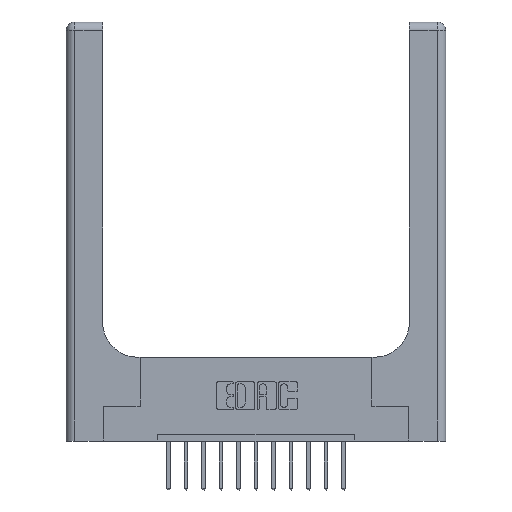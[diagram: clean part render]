
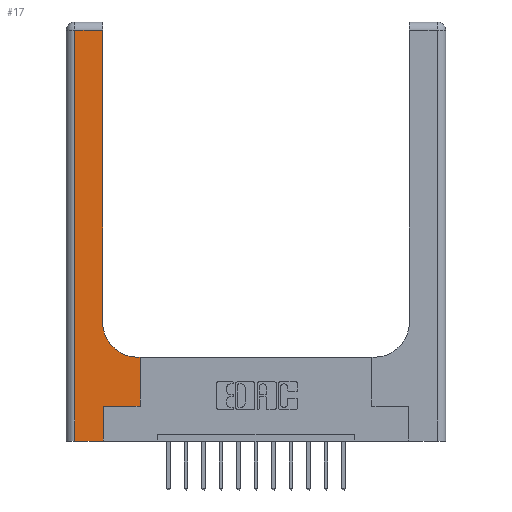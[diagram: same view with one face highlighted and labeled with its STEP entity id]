
A CAD part, top view. The second image highlights one B-rep face of the part: STEP entity #17.
In plain terms, the highlighted planar face has unit normal (0, 0, 1).
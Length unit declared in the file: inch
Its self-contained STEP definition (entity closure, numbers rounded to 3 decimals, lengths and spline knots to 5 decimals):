
#17 = ADVANCED_FACE ( 'NONE', ( #8297 ), #3548, .F. ) ;
#276 = DIRECTION ( 'NONE',  ( -1., 0., 0. ) ) ;
#366 = DIRECTION ( 'NONE',  ( 0., 0., -1. ) ) ;
#602 = CIRCLE ( 'NONE', #13419, 0.25 ) ;
#658 = EDGE_CURVE ( 'NONE', #3777, #8565, #3033, .T. ) ;
#773 = DIRECTION ( 'NONE',  ( 0., -1., 0. ) ) ;
#930 = CARTESIAN_POINT ( 'NONE',  ( 0.06, 3., 0.37 ) ) ;
#1183 = ORIENTED_EDGE ( 'NONE', *, *, #7869, .T. ) ;
#1804 = LINE ( 'NONE', #13499, #14296 ) ;
#2345 = VECTOR ( 'NONE', #6904, 39.37008 ) ;
#2605 = VERTEX_POINT ( 'NONE', #16104 ) ;
#3033 = LINE ( 'NONE', #5393, #12925 ) ;
#3062 = LINE ( 'NONE', #13280, #2345 ) ;
#3382 = CARTESIAN_POINT ( 'NONE',  ( 0.265, 0., 0.37 ) ) ;
#3548 = PLANE ( 'NONE',  #11623 ) ;
#3777 = VERTEX_POINT ( 'NONE', #10324 ) ;
#3951 = EDGE_CURVE ( 'NONE', #8565, #15572, #9876, .T. ) ;
#4087 = VECTOR ( 'NONE', #276, 39.37008 ) ;
#4134 = VERTEX_POINT ( 'NONE', #13182 ) ;
#4283 = CARTESIAN_POINT ( 'NONE',  ( 0.26, 0.6, 0.37 ) ) ;
#4642 = ORIENTED_EDGE ( 'NONE', *, *, #14886, .T. ) ;
#4965 = CARTESIAN_POINT ( 'NONE',  ( 0.528, 0.25, 0.37 ) ) ;
#5393 = CARTESIAN_POINT ( 'NONE',  ( 0.265, 0.25, 0.37 ) ) ;
#5454 = CARTESIAN_POINT ( 'NONE',  ( 0.528, 0.25, 0.37 ) ) ;
#5489 = DIRECTION ( 'NONE',  ( 1., 0., 0. ) ) ;
#5924 = ORIENTED_EDGE ( 'NONE', *, *, #7229, .T. ) ;
#6159 = ORIENTED_EDGE ( 'NONE', *, *, #16539, .T. ) ;
#6294 = VERTEX_POINT ( 'NONE', #13124 ) ;
#6359 = VECTOR ( 'NONE', #773, 39.37008 ) ;
#6543 = ORIENTED_EDGE ( 'NONE', *, *, #11967, .T. ) ;
#6786 = DIRECTION ( 'NONE',  ( -1., 0., 0. ) ) ;
#6896 = DIRECTION ( 'NONE',  ( 0., 1., 0. ) ) ;
#6904 = DIRECTION ( 'NONE',  ( 1., 0., 0. ) ) ;
#7229 = EDGE_CURVE ( 'NONE', #14893, #3777, #13504, .T. ) ;
#7474 = VECTOR ( 'NONE', #9756, 39.37008 ) ;
#7869 = EDGE_CURVE ( 'NONE', #15572, #4134, #12845, .T. ) ;
#8044 = LINE ( 'NONE', #11935, #4087 ) ;
#8297 = FACE_OUTER_BOUND ( 'NONE', #9561, .T. ) ;
#8565 = VERTEX_POINT ( 'NONE', #5454 ) ;
#8634 = DIRECTION ( 'NONE',  ( -1., 0., 0. ) ) ;
#8945 = CARTESIAN_POINT ( 'NONE',  ( 0.06, 0., 0.37 ) ) ;
#8964 = ORIENTED_EDGE ( 'NONE', *, *, #658, .T. ) ;
#9164 = CARTESIAN_POINT ( 'NONE',  ( 0.51, 0.85, 0.37 ) ) ;
#9298 = VERTEX_POINT ( 'NONE', #11105 ) ;
#9561 = EDGE_LOOP ( 'NONE', ( #6543, #6159, #4642, #15254, #5924, #8964, #10467, #1183, #13441 ) ) ;
#9756 = DIRECTION ( 'NONE',  ( 0., 1., 0. ) ) ;
#9825 = CARTESIAN_POINT ( 'NONE',  ( 0., 3., 0.37 ) ) ;
#9876 = LINE ( 'NONE', #4965, #14426 ) ;
#10196 = VERTEX_POINT ( 'NONE', #8945 ) ;
#10324 = CARTESIAN_POINT ( 'NONE',  ( 0.265, 0.25, 0.37 ) ) ;
#10467 = ORIENTED_EDGE ( 'NONE', *, *, #3951, .T. ) ;
#11080 = LINE ( 'NONE', #930, #6359 ) ;
#11105 = CARTESIAN_POINT ( 'NONE',  ( 0.26, 2.94, 0.37 ) ) ;
#11623 = AXIS2_PLACEMENT_3D ( 'NONE', #9825, #14974, #8634 ) ;
#11935 = CARTESIAN_POINT ( 'NONE',  ( 0., 2.94, 0.37 ) ) ;
#11967 = EDGE_CURVE ( 'NONE', #6294, #9298, #1804, .T. ) ;
#12845 = LINE ( 'NONE', #4283, #15037 ) ;
#12925 = VECTOR ( 'NONE', #13101, 39.37008 ) ;
#13101 = DIRECTION ( 'NONE',  ( 1., 0., 0. ) ) ;
#13124 = CARTESIAN_POINT ( 'NONE',  ( 0.26, 0.85, 0.37 ) ) ;
#13182 = CARTESIAN_POINT ( 'NONE',  ( 0.51, 0.6, 0.37 ) ) ;
#13247 = EDGE_CURVE ( 'NONE', #10196, #14893, #3062, .T. ) ;
#13280 = CARTESIAN_POINT ( 'NONE',  ( 0., 0., 0.37 ) ) ;
#13419 = AXIS2_PLACEMENT_3D ( 'NONE', #9164, #366, #5489 ) ;
#13441 = ORIENTED_EDGE ( 'NONE', *, *, #16541, .T. ) ;
#13499 = CARTESIAN_POINT ( 'NONE',  ( 0.26, 3., 0.37 ) ) ;
#13504 = LINE ( 'NONE', #13659, #7474 ) ;
#13659 = CARTESIAN_POINT ( 'NONE',  ( 0.265, 0., 0.37 ) ) ;
#14296 = VECTOR ( 'NONE', #6896, 39.37008 ) ;
#14426 = VECTOR ( 'NONE', #15484, 39.37008 ) ;
#14886 = EDGE_CURVE ( 'NONE', #2605, #10196, #11080, .T. ) ;
#14893 = VERTEX_POINT ( 'NONE', #3382 ) ;
#14974 = DIRECTION ( 'NONE',  ( 0., 0., -1. ) ) ;
#15037 = VECTOR ( 'NONE', #6786, 39.37008 ) ;
#15254 = ORIENTED_EDGE ( 'NONE', *, *, #13247, .T. ) ;
#15484 = DIRECTION ( 'NONE',  ( 0., 1., 0. ) ) ;
#15572 = VERTEX_POINT ( 'NONE', #16253 ) ;
#16104 = CARTESIAN_POINT ( 'NONE',  ( 0.06, 2.94, 0.37 ) ) ;
#16253 = CARTESIAN_POINT ( 'NONE',  ( 0.528, 0.6, 0.37 ) ) ;
#16539 = EDGE_CURVE ( 'NONE', #9298, #2605, #8044, .T. ) ;
#16541 = EDGE_CURVE ( 'NONE', #4134, #6294, #602, .T. ) ;
